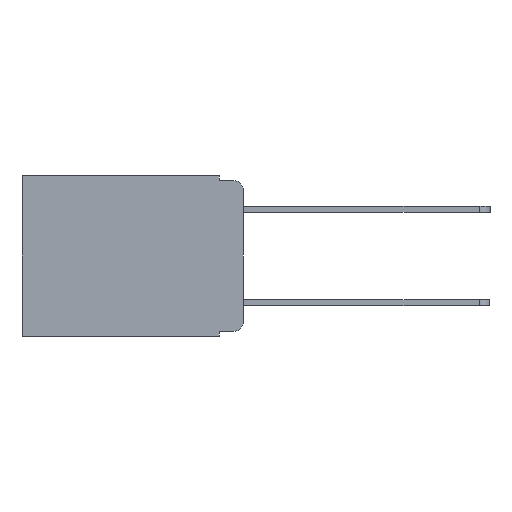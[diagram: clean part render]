
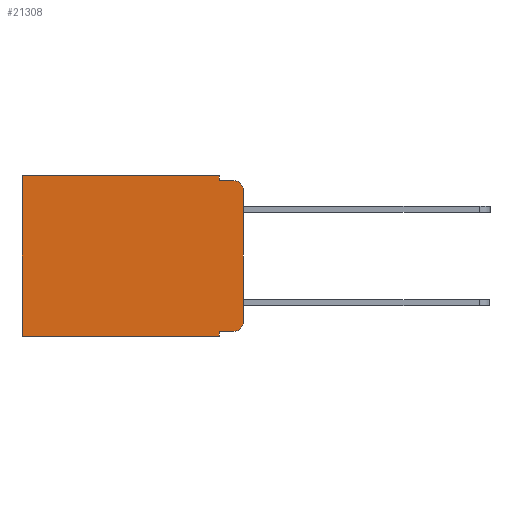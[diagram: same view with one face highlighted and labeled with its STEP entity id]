
A CAD part, left-side view. The second image highlights one B-rep face of the part: STEP entity #21308.
In plain terms, the highlighted planar face has unit normal (-1, 0, 0).
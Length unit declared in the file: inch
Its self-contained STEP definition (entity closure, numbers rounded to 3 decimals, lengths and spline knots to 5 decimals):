
#150 = ORIENTED_EDGE ( 'NONE', *, *, #13604, .T. ) ;
#269 = CIRCLE ( 'NONE', #19956, 0.02 ) ;
#322 = LINE ( 'NONE', #13869, #4516 ) ;
#455 = ORIENTED_EDGE ( 'NONE', *, *, #9913, .F. ) ;
#499 = VERTEX_POINT ( 'NONE', #6871 ) ;
#731 = DIRECTION ( 'NONE',  ( 1., 0., 0. ) ) ;
#1073 = EDGE_LOOP ( 'NONE', ( #4623, #150, #455, #2721, #19731, #3815, #5714, #8399, #11310, #14657 ) ) ;
#1777 = DIRECTION ( 'NONE',  ( 0., 1., 0. ) ) ;
#2646 = EDGE_CURVE ( 'NONE', #3853, #499, #16536, .T. ) ;
#2721 = ORIENTED_EDGE ( 'NONE', *, *, #18321, .F. ) ;
#2859 = VECTOR ( 'NONE', #15336, 39.37008 ) ;
#2953 = EDGE_CURVE ( 'NONE', #6783, #499, #16275, .T. ) ;
#3092 = EDGE_CURVE ( 'NONE', #6439, #6783, #322, .T. ) ;
#3455 = DIRECTION ( 'NONE',  ( 0., 0., -1. ) ) ;
#3528 = CARTESIAN_POINT ( 'NONE',  ( 0.298, 0.02, -0.01 ) ) ;
#3669 = CARTESIAN_POINT ( 'NONE',  ( 0.298, 0.051, -0.01 ) ) ;
#3815 = ORIENTED_EDGE ( 'NONE', *, *, #2953, .T. ) ;
#3853 = VERTEX_POINT ( 'NONE', #13077 ) ;
#3883 = FACE_OUTER_BOUND ( 'NONE', #1073, .T. ) ;
#4140 = CARTESIAN_POINT ( 'NONE',  ( 0.298, 0., 0. ) ) ;
#4377 = CARTESIAN_POINT ( 'NONE',  ( 0.298, 0.473, 0. ) ) ;
#4507 = LINE ( 'NONE', #7659, #13080 ) ;
#4516 = VECTOR ( 'NONE', #1777, 39.37008 ) ;
#4556 = EDGE_CURVE ( 'NONE', #14593, #15749, #12804, .T. ) ;
#4623 = ORIENTED_EDGE ( 'NONE', *, *, #4556, .F. ) ;
#5355 = VERTEX_POINT ( 'NONE', #8635 ) ;
#5612 = AXIS2_PLACEMENT_3D ( 'NONE', #21134, #731, #12871 ) ;
#5714 = ORIENTED_EDGE ( 'NONE', *, *, #2646, .F. ) ;
#5867 = LINE ( 'NONE', #20890, #9889 ) ;
#5989 = VERTEX_POINT ( 'NONE', #18374 ) ;
#6439 = VERTEX_POINT ( 'NONE', #14465 ) ;
#6626 = CARTESIAN_POINT ( 'NONE',  ( 0.298, 0., -0.313 ) ) ;
#6761 = LINE ( 'NONE', #3669, #15298 ) ;
#6783 = VERTEX_POINT ( 'NONE', #9797 ) ;
#6871 = CARTESIAN_POINT ( 'NONE',  ( 0.298, 0.473, -0.343 ) ) ;
#7255 = CARTESIAN_POINT ( 'NONE',  ( 0.298, 0.02, -0.313 ) ) ;
#7659 = CARTESIAN_POINT ( 'NONE',  ( 0.298, 0.051, 0. ) ) ;
#8399 = ORIENTED_EDGE ( 'NONE', *, *, #11950, .F. ) ;
#8635 = CARTESIAN_POINT ( 'NONE',  ( 0.298, 0.051, -0.333 ) ) ;
#8911 = LINE ( 'NONE', #19642, #12881 ) ;
#8984 = DIRECTION ( 'NONE',  ( 0., 0., -1. ) ) ;
#9671 = CARTESIAN_POINT ( 'NONE',  ( 0.298, 0.051, -0.01 ) ) ;
#9797 = CARTESIAN_POINT ( 'NONE',  ( 0.298, 0.473, 0. ) ) ;
#9889 = VECTOR ( 'NONE', #15956, 39.37008 ) ;
#9913 = EDGE_CURVE ( 'NONE', #16735, #11783, #6761, .T. ) ;
#10349 = CARTESIAN_POINT ( 'NONE',  ( 0.298, 0.02, -0.03 ) ) ;
#11310 = ORIENTED_EDGE ( 'NONE', *, *, #19579, .T. ) ;
#11414 = DIRECTION ( 'NONE',  ( 0., -1., 0. ) ) ;
#11783 = VERTEX_POINT ( 'NONE', #3528 ) ;
#11950 = EDGE_CURVE ( 'NONE', #5355, #3853, #5867, .T. ) ;
#12050 = DIRECTION ( 'NONE',  ( 0., 0., -1. ) ) ;
#12278 = VECTOR ( 'NONE', #3455, 39.37008 ) ;
#12314 = VECTOR ( 'NONE', #14639, 39.37008 ) ;
#12804 = LINE ( 'NONE', #4140, #12278 ) ;
#12871 = DIRECTION ( 'NONE',  ( 0., 0., -1. ) ) ;
#12881 = VECTOR ( 'NONE', #11414, 39.37008 ) ;
#13077 = CARTESIAN_POINT ( 'NONE',  ( 0.298, 0.051, -0.343 ) ) ;
#13080 = VECTOR ( 'NONE', #17763, 39.37008 ) ;
#13604 = EDGE_CURVE ( 'NONE', #14593, #11783, #14882, .T. ) ;
#13869 = CARTESIAN_POINT ( 'NONE',  ( 0.298, 0., 0. ) ) ;
#13909 = AXIS2_PLACEMENT_3D ( 'NONE', #10349, #21964, #12050 ) ;
#14465 = CARTESIAN_POINT ( 'NONE',  ( 0.298, 0.051, 0. ) ) ;
#14593 = VERTEX_POINT ( 'NONE', #21977 ) ;
#14639 = DIRECTION ( 'NONE',  ( 0., 0., -1. ) ) ;
#14657 = ORIENTED_EDGE ( 'NONE', *, *, #18791, .T. ) ;
#14882 = CIRCLE ( 'NONE', #13909, 0.02 ) ;
#15298 = VECTOR ( 'NONE', #18965, 39.37008 ) ;
#15336 = DIRECTION ( 'NONE',  ( 0., 1., 0. ) ) ;
#15749 = VERTEX_POINT ( 'NONE', #6626 ) ;
#15956 = DIRECTION ( 'NONE',  ( 0., 0., -1. ) ) ;
#16275 = LINE ( 'NONE', #4377, #12314 ) ;
#16536 = LINE ( 'NONE', #17004, #2859 ) ;
#16735 = VERTEX_POINT ( 'NONE', #9671 ) ;
#17004 = CARTESIAN_POINT ( 'NONE',  ( 0.298, 0., -0.343 ) ) ;
#17763 = DIRECTION ( 'NONE',  ( 0., 0., -1. ) ) ;
#18321 = EDGE_CURVE ( 'NONE', #6439, #16735, #4507, .T. ) ;
#18374 = CARTESIAN_POINT ( 'NONE',  ( 0.298, 0.02, -0.333 ) ) ;
#18791 = EDGE_CURVE ( 'NONE', #5989, #15749, #269, .T. ) ;
#18965 = DIRECTION ( 'NONE',  ( 0., -1., 0. ) ) ;
#19021 = DIRECTION ( 'NONE',  ( -1., 0., 0. ) ) ;
#19500 = PLANE ( 'NONE',  #5612 ) ;
#19579 = EDGE_CURVE ( 'NONE', #5355, #5989, #8911, .T. ) ;
#19642 = CARTESIAN_POINT ( 'NONE',  ( 0.298, 0.051, -0.333 ) ) ;
#19731 = ORIENTED_EDGE ( 'NONE', *, *, #3092, .T. ) ;
#19956 = AXIS2_PLACEMENT_3D ( 'NONE', #7255, #19021, #8984 ) ;
#20890 = CARTESIAN_POINT ( 'NONE',  ( 0.298, 0.051, 0. ) ) ;
#21134 = CARTESIAN_POINT ( 'NONE',  ( 0.298, 0., 0. ) ) ;
#21308 = ADVANCED_FACE ( 'NONE', ( #3883 ), #19500, .F. ) ;
#21964 = DIRECTION ( 'NONE',  ( -1., 0., 0. ) ) ;
#21977 = CARTESIAN_POINT ( 'NONE',  ( 0.298, 0., -0.03 ) ) ;
